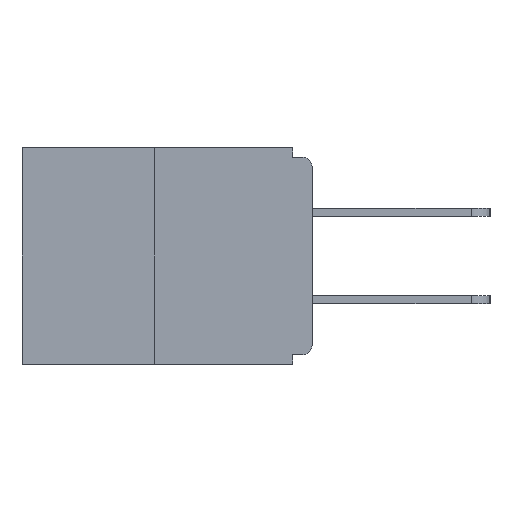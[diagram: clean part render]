
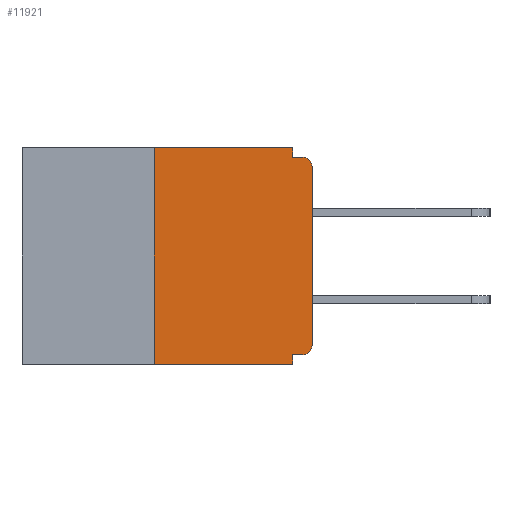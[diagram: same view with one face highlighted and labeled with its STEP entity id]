
A CAD part, left-side view. The second image highlights one B-rep face of the part: STEP entity #11921.
In plain terms, the highlighted planar face has unit normal (-1, 0, 0).
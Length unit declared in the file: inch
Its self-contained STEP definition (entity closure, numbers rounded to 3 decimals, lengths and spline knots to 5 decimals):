
#326 = EDGE_CURVE ( 'NONE', #15125, #7207, #9840, .T. ) ;
#536 = LINE ( 'NONE', #1678, #15592 ) ;
#597 = CARTESIAN_POINT ( 'NONE',  ( 0., 0.25, 0. ) ) ;
#651 = ORIENTED_EDGE ( 'NONE', *, *, #326, .T. ) ;
#910 = VECTOR ( 'NONE', #11950, 39.37008 ) ;
#951 = VERTEX_POINT ( 'NONE', #7990 ) ;
#1079 = PLANE ( 'NONE',  #17701 ) ;
#1678 = CARTESIAN_POINT ( 'NONE',  ( 0., 0.46, -0.343 ) ) ;
#2054 = ORIENTED_EDGE ( 'NONE', *, *, #3723, .F. ) ;
#2071 = VERTEX_POINT ( 'NONE', #4474 ) ;
#2126 = ORIENTED_EDGE ( 'NONE', *, *, #22141, .T. ) ;
#2200 = VECTOR ( 'NONE', #14126, 39.37008 ) ;
#2307 = DIRECTION ( 'NONE',  ( -1., 0., 0. ) ) ;
#2634 = CARTESIAN_POINT ( 'NONE',  ( 0., 0.015, -0.313 ) ) ;
#2994 = VERTEX_POINT ( 'NONE', #21581 ) ;
#3008 = CARTESIAN_POINT ( 'NONE',  ( 0., 0.25, -0.343 ) ) ;
#3253 = VECTOR ( 'NONE', #5520, 39.37008 ) ;
#3393 = ORIENTED_EDGE ( 'NONE', *, *, #20016, .F. ) ;
#3443 = CARTESIAN_POINT ( 'NONE',  ( 0., 0., -0.03 ) ) ;
#3723 = EDGE_CURVE ( 'NONE', #2071, #25213, #6509, .T. ) ;
#4317 = VECTOR ( 'NONE', #9810, 39.37008 ) ;
#4474 = CARTESIAN_POINT ( 'NONE',  ( 0., 0.25, 0. ) ) ;
#4601 = EDGE_CURVE ( 'NONE', #15125, #951, #9839, .T. ) ;
#4713 = VERTEX_POINT ( 'NONE', #3443 ) ;
#5391 = DIRECTION ( 'NONE',  ( 0., -1., 0. ) ) ;
#5520 = DIRECTION ( 'NONE',  ( 0., -1., 0. ) ) ;
#5699 = EDGE_CURVE ( 'NONE', #25213, #2994, #9159, .T. ) ;
#6161 = VECTOR ( 'NONE', #8046, 39.37008 ) ;
#6509 = LINE ( 'NONE', #13200, #12004 ) ;
#7157 = VERTEX_POINT ( 'NONE', #12766 ) ;
#7207 = VERTEX_POINT ( 'NONE', #22557 ) ;
#7250 = DIRECTION ( 'NONE',  ( 0., -1., 0. ) ) ;
#7682 = CARTESIAN_POINT ( 'NONE',  ( 0., 0., -0.015 ) ) ;
#7990 = CARTESIAN_POINT ( 'NONE',  ( 0., 0.031, -0.328 ) ) ;
#8046 = DIRECTION ( 'NONE',  ( 0., 0., 1. ) ) ;
#8145 = ORIENTED_EDGE ( 'NONE', *, *, #20799, .T. ) ;
#8323 = AXIS2_PLACEMENT_3D ( 'NONE', #2634, #2307, #20401 ) ;
#9141 = CARTESIAN_POINT ( 'NONE',  ( 0., 0.031, -0.343 ) ) ;
#9159 = LINE ( 'NONE', #14171, #18378 ) ;
#9771 = CARTESIAN_POINT ( 'NONE',  ( 0., 0.031, 0. ) ) ;
#9794 = EDGE_CURVE ( 'NONE', #951, #16444, #24972, .T. ) ;
#9810 = DIRECTION ( 'NONE',  ( 0., 0., -1. ) ) ;
#9839 = LINE ( 'NONE', #11870, #910 ) ;
#9840 = CIRCLE ( 'NONE', #8323, 0.015 ) ;
#10085 = CARTESIAN_POINT ( 'NONE',  ( 0., 0.015, -0.328 ) ) ;
#10477 = LINE ( 'NONE', #597, #2200 ) ;
#11063 = DIRECTION ( 'NONE',  ( -1., 0., 0. ) ) ;
#11717 = ORIENTED_EDGE ( 'NONE', *, *, #5699, .F. ) ;
#11870 = CARTESIAN_POINT ( 'NONE',  ( 0., 0., -0.328 ) ) ;
#11921 = ADVANCED_FACE ( 'NONE', ( #13364 ), #1079, .F. ) ;
#11950 = DIRECTION ( 'NONE',  ( 0., 1., 0. ) ) ;
#11974 = ORIENTED_EDGE ( 'NONE', *, *, #23007, .F. ) ;
#12004 = VECTOR ( 'NONE', #7250, 39.37008 ) ;
#12760 = EDGE_CURVE ( 'NONE', #4713, #7157, #19297, .T. ) ;
#12766 = CARTESIAN_POINT ( 'NONE',  ( 0., 0.015, -0.015 ) ) ;
#13142 = DIRECTION ( 'NONE',  ( 0., 0., -1. ) ) ;
#13161 = LINE ( 'NONE', #17731, #6161 ) ;
#13200 = CARTESIAN_POINT ( 'NONE',  ( 0., 0.46, 0. ) ) ;
#13364 = FACE_OUTER_BOUND ( 'NONE', #24288, .T. ) ;
#14126 = DIRECTION ( 'NONE',  ( 0., 0., 1. ) ) ;
#14171 = CARTESIAN_POINT ( 'NONE',  ( 0., 0.031, 0. ) ) ;
#14280 = VERTEX_POINT ( 'NONE', #3008 ) ;
#14889 = ORIENTED_EDGE ( 'NONE', *, *, #4601, .F. ) ;
#14986 = CARTESIAN_POINT ( 'NONE',  ( 0., 0.015, -0.03 ) ) ;
#15125 = VERTEX_POINT ( 'NONE', #10085 ) ;
#15592 = VECTOR ( 'NONE', #5391, 39.37008 ) ;
#16444 = VERTEX_POINT ( 'NONE', #9141 ) ;
#17464 = ORIENTED_EDGE ( 'NONE', *, *, #12760, .T. ) ;
#17689 = LINE ( 'NONE', #7682, #3253 ) ;
#17701 = AXIS2_PLACEMENT_3D ( 'NONE', #25035, #19070, #13142 ) ;
#17731 = CARTESIAN_POINT ( 'NONE',  ( 0., 0., 0. ) ) ;
#17774 = CARTESIAN_POINT ( 'NONE',  ( 0., 0.031, -0.343 ) ) ;
#18378 = VECTOR ( 'NONE', #22089, 39.37008 ) ;
#19070 = DIRECTION ( 'NONE',  ( 1., 0., 0. ) ) ;
#19297 = CIRCLE ( 'NONE', #23879, 0.015 ) ;
#20016 = EDGE_CURVE ( 'NONE', #14280, #2071, #10477, .T. ) ;
#20401 = DIRECTION ( 'NONE',  ( 0., 0., -1. ) ) ;
#20799 = EDGE_CURVE ( 'NONE', #7207, #4713, #13161, .T. ) ;
#21581 = CARTESIAN_POINT ( 'NONE',  ( 0., 0.031, -0.015 ) ) ;
#22089 = DIRECTION ( 'NONE',  ( 0., 0., -1. ) ) ;
#22141 = EDGE_CURVE ( 'NONE', #14280, #16444, #536, .T. ) ;
#22557 = CARTESIAN_POINT ( 'NONE',  ( 0., 0., -0.313 ) ) ;
#23007 = EDGE_CURVE ( 'NONE', #2994, #7157, #17689, .T. ) ;
#23879 = AXIS2_PLACEMENT_3D ( 'NONE', #14986, #11063, #24791 ) ;
#24288 = EDGE_LOOP ( 'NONE', ( #2054, #3393, #2126, #24409, #14889, #651, #8145, #17464, #11974, #11717 ) ) ;
#24409 = ORIENTED_EDGE ( 'NONE', *, *, #9794, .F. ) ;
#24791 = DIRECTION ( 'NONE',  ( 0., 0., -1. ) ) ;
#24972 = LINE ( 'NONE', #17774, #4317 ) ;
#25035 = CARTESIAN_POINT ( 'NONE',  ( 0., 0.46, 0. ) ) ;
#25213 = VERTEX_POINT ( 'NONE', #9771 ) ;
